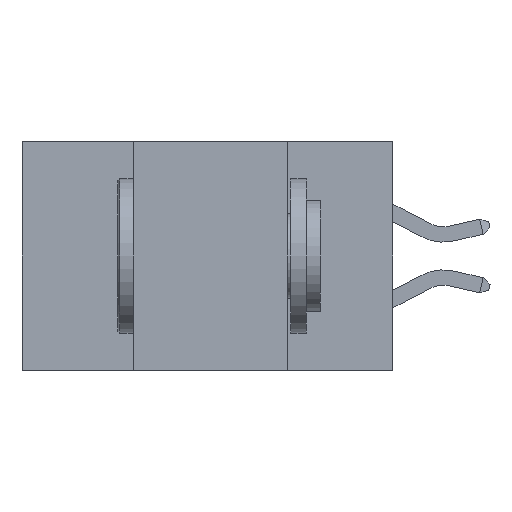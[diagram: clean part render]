
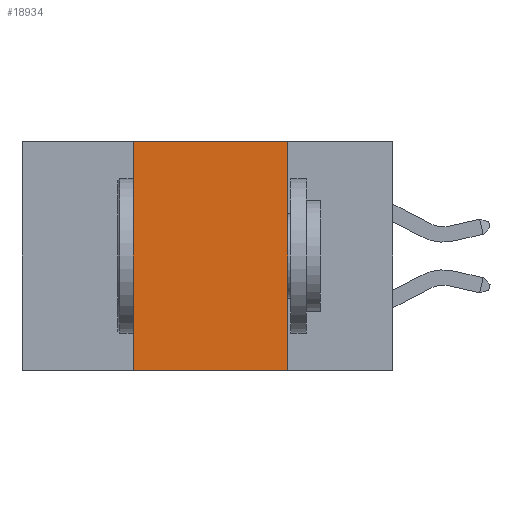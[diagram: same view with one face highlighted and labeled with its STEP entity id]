
A CAD part, left-side view. The second image highlights one B-rep face of the part: STEP entity #18934.
In plain terms, the highlighted planar face has unit normal (-1, 0, 0).
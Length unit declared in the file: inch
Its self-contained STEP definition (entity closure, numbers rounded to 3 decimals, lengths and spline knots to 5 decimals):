
#301 = ORIENTED_EDGE ( 'NONE', *, *, #8249, .F. ) ;
#464 = AXIS2_PLACEMENT_3D ( 'NONE', #2637, #20349, #7314 ) ;
#1300 = CARTESIAN_POINT ( 'NONE',  ( 0., 0.42, 0. ) ) ;
#1343 = EDGE_CURVE ( 'NONE', #13027, #13313, #20275, .T. ) ;
#1573 = FACE_OUTER_BOUND ( 'NONE', #5487, .T. ) ;
#2210 = ORIENTED_EDGE ( 'NONE', *, *, #1343, .F. ) ;
#2637 = CARTESIAN_POINT ( 'NONE',  ( 0., 0.6, 0. ) ) ;
#3941 = ORIENTED_EDGE ( 'NONE', *, *, #7095, .F. ) ;
#5285 = DIRECTION ( 'NONE',  ( 0., -1., 0. ) ) ;
#5487 = EDGE_LOOP ( 'NONE', ( #2210, #3941, #301, #16238 ) ) ;
#6066 = LINE ( 'NONE', #20227, #9854 ) ;
#6486 = VECTOR ( 'NONE', #5285, 39.37008 ) ;
#7080 = LINE ( 'NONE', #1300, #10648 ) ;
#7095 = EDGE_CURVE ( 'NONE', #15914, #13027, #6066, .T. ) ;
#7314 = DIRECTION ( 'NONE',  ( 0., 0., -1. ) ) ;
#7323 = VERTEX_POINT ( 'NONE', #13199 ) ;
#8249 = EDGE_CURVE ( 'NONE', #7323, #15914, #7080, .T. ) ;
#8700 = CARTESIAN_POINT ( 'NONE',  ( 0., 0.17, 0. ) ) ;
#9854 = VECTOR ( 'NONE', #20231, 39.37008 ) ;
#10590 = CARTESIAN_POINT ( 'NONE',  ( 0., 0.17, -0.37 ) ) ;
#10648 = VECTOR ( 'NONE', #12625, 39.37008 ) ;
#10797 = LINE ( 'NONE', #18115, #6486 ) ;
#12172 = CARTESIAN_POINT ( 'NONE',  ( 0., 0.17, 0. ) ) ;
#12625 = DIRECTION ( 'NONE',  ( 0., 0., 1. ) ) ;
#13027 = VERTEX_POINT ( 'NONE', #12172 ) ;
#13199 = CARTESIAN_POINT ( 'NONE',  ( 0., 0.42, -0.37 ) ) ;
#13313 = VERTEX_POINT ( 'NONE', #10590 ) ;
#14770 = CARTESIAN_POINT ( 'NONE',  ( 0., 0.42, 0. ) ) ;
#15743 = VECTOR ( 'NONE', #20061, 39.37008 ) ;
#15914 = VERTEX_POINT ( 'NONE', #14770 ) ;
#16104 = EDGE_CURVE ( 'NONE', #7323, #13313, #10797, .T. ) ;
#16238 = ORIENTED_EDGE ( 'NONE', *, *, #16104, .T. ) ;
#18115 = CARTESIAN_POINT ( 'NONE',  ( 0., 0.6, -0.37 ) ) ;
#18747 = PLANE ( 'NONE',  #464 ) ;
#18934 = ADVANCED_FACE ( 'NONE', ( #1573 ), #18747, .F. ) ;
#20061 = DIRECTION ( 'NONE',  ( 0., 0., -1. ) ) ;
#20227 = CARTESIAN_POINT ( 'NONE',  ( 0., 0.6, 0. ) ) ;
#20231 = DIRECTION ( 'NONE',  ( 0., -1., 0. ) ) ;
#20275 = LINE ( 'NONE', #8700, #15743 ) ;
#20349 = DIRECTION ( 'NONE',  ( 1., 0., 0. ) ) ;
